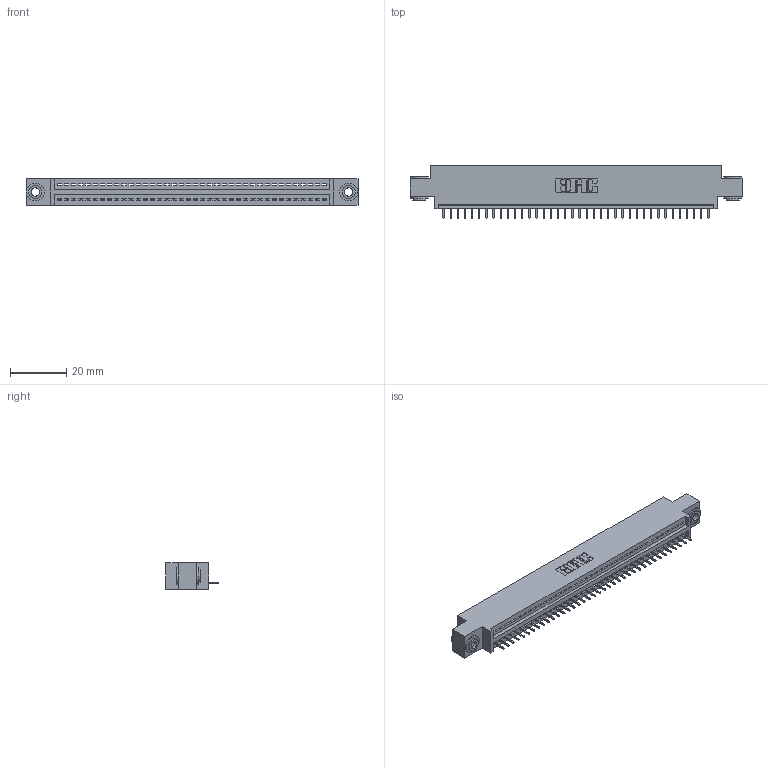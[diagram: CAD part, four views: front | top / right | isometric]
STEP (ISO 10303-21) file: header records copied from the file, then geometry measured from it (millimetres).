
FILE_DESCRIPTION (( 'STEP AP203' ), '1' );
FILE_NAME ('895-038-525-603.STEP', '2020-09-26T01:51:22', ( '' ), ( '' ), 'SwSTEP 2.0', 'SolidWorks 2020', '' );
FILE_SCHEMA (( 'CONFIG_CONTROL_DESIGN' ));
Length unit declared in the file: inch
Products named in the file (4): 345-292-001_345-293-125; 845 Part_0.170 Offset - 0.156 Dia-TH; 895-038-525-603; 345-250-002_345-250-002-102
Assembly tree (41 placements, depth 2):
  895-038-525-603
    845 Part_0.170 Offset - 0.156 Dia-TH
    345-292-001_345-293-125  x38
    345-250-002_345-250-002-102  x2
Bounding box: 117.73 x 18.72 x 9.4 mm (x, y, z)
Volume: 10900.1 mm3; surface area: 14254.5 mm2
Topology: 41 solids, 41 shells, 2524 faces, 7269 edges, 4690 vertices
Faces by surface type: plane 1842, cylinder 674, cone 8
Entity records: 29994 total; most frequent: CARTESIAN_POINT 5173, ORIENTED_EDGE 5138, DIRECTION 4555, EDGE_CURVE 2569, LINE 2265, VECTOR 2265, VERTEX_POINT 1706, AXIS2_PLACEMENT_3D 1145
